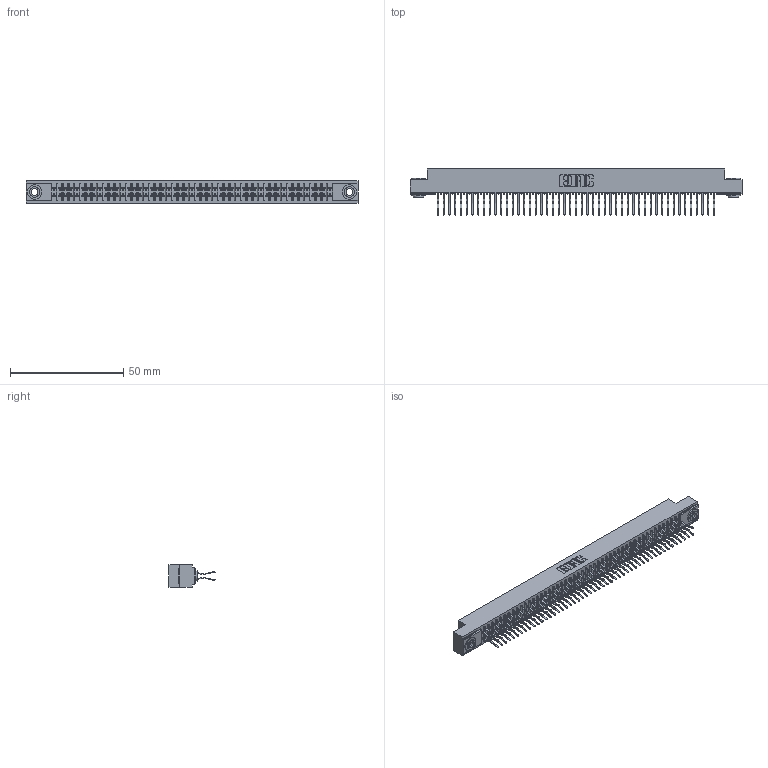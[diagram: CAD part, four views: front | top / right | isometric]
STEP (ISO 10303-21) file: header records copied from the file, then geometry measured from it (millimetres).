
FILE_DESCRIPTION (( 'STEP AP203' ), '1' );
FILE_NAME ('391-098-560-203.STEP', '2018-08-09T19:16:31', ( '' ), ( '' ), 'SwSTEP 2.0', 'SolidWorks 2016', '' );
FILE_SCHEMA (( 'CONFIG_CONTROL_DESIGN' ));
Length unit declared in the file: inch
Products named in the file (4): 341-292-001_341-292-160; 345-250-002_345-250-002-102; 391-098-560-203; 341 Part_.156 (3.96) Dia Mounting Holes
Assembly tree (101 placements, depth 2):
  391-098-560-203
    341 Part_.156 (3.96) Dia Mounting Holes
    341-292-001_341-292-160  x98
    345-250-002_345-250-002-102  x2
Bounding box: 146.69 x 20.37 x 10.16 mm (x, y, z)
Volume: 10936.7 mm3; surface area: 20604.7 mm2
Topology: 101 solids, 101 shells, 7028 faces, 20371 edges, 13214 vertices
Faces by surface type: plane 4012, cylinder 2812, sphere 100, torus 96, cone 8
Entity records: 59573 total; most frequent: CARTESIAN_POINT 9884, ORIENTED_EDGE 9814, DIRECTION 9607, EDGE_CURVE 4907, VECTOR 3957, LINE 3957, VERTEX_POINT 3102, AXIS2_PLACEMENT_3D 2825
